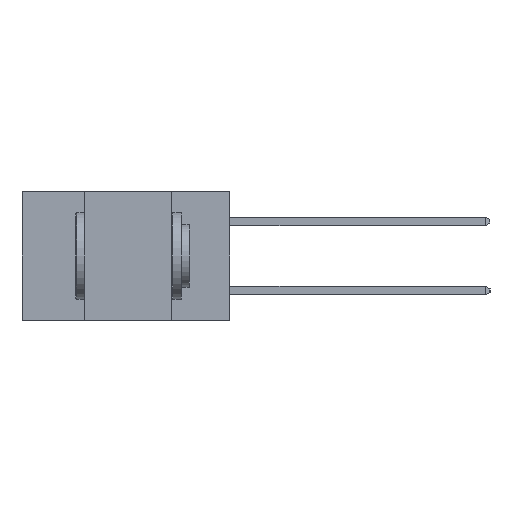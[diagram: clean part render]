
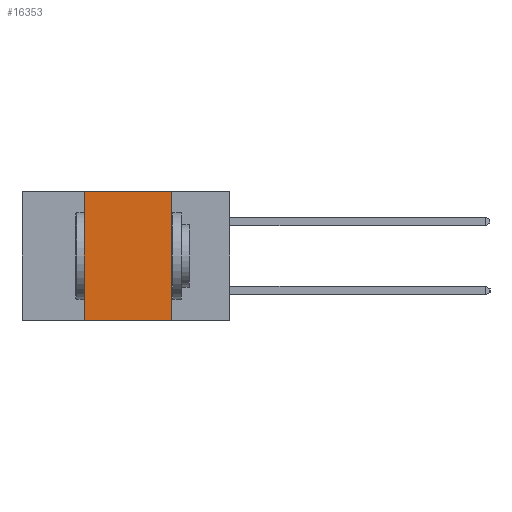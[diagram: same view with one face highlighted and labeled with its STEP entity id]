
A CAD part, left-side view. The second image highlights one B-rep face of the part: STEP entity #16353.
In plain terms, the highlighted planar face has unit normal (-1, 0, 0).
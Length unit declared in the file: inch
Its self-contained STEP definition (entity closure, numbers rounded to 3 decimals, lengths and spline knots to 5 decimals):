
#102 = VECTOR ( 'NONE', #20577, 39.37008 ) ;
#671 = ORIENTED_EDGE ( 'NONE', *, *, #18440, .T. ) ;
#1120 = DIRECTION ( 'NONE',  ( 0., -1., 0. ) ) ;
#3769 = ORIENTED_EDGE ( 'NONE', *, *, #21884, .F. ) ;
#5909 = FACE_OUTER_BOUND ( 'NONE', #11391, .T. ) ;
#6628 = CARTESIAN_POINT ( 'NONE',  ( 0., 0.6, 0. ) ) ;
#6913 = DIRECTION ( 'NONE',  ( 0., 0., 1. ) ) ;
#7944 = VERTEX_POINT ( 'NONE', #11834 ) ;
#8333 = VERTEX_POINT ( 'NONE', #8400 ) ;
#8400 = CARTESIAN_POINT ( 'NONE',  ( 0., 0.17, -0.37 ) ) ;
#8561 = VECTOR ( 'NONE', #1120, 39.37008 ) ;
#8564 = CARTESIAN_POINT ( 'NONE',  ( 0., 0.17, -0.37 ) ) ;
#9025 = ORIENTED_EDGE ( 'NONE', *, *, #19572, .F. ) ;
#9499 = DIRECTION ( 'NONE',  ( 0., 0., -1. ) ) ;
#11143 = PLANE ( 'NONE',  #19806 ) ;
#11391 = EDGE_LOOP ( 'NONE', ( #3769, #22169, #9025, #671 ) ) ;
#11834 = CARTESIAN_POINT ( 'NONE',  ( 0., 0.42, 0. ) ) ;
#12068 = LINE ( 'NONE', #21934, #8561 ) ;
#12415 = CARTESIAN_POINT ( 'NONE',  ( 0., 0.17, 0. ) ) ;
#12537 = LINE ( 'NONE', #13794, #16591 ) ;
#12584 = VERTEX_POINT ( 'NONE', #12415 ) ;
#13794 = CARTESIAN_POINT ( 'NONE',  ( 0., 0.42, -0.37 ) ) ;
#14913 = LINE ( 'NONE', #6628, #20034 ) ;
#16346 = CARTESIAN_POINT ( 'NONE',  ( 0., 0.6, 0. ) ) ;
#16353 = ADVANCED_FACE ( 'NONE', ( #5909 ), #11143, .F. ) ;
#16591 = VECTOR ( 'NONE', #6913, 39.37008 ) ;
#16983 = DIRECTION ( 'NONE',  ( 0., -1., 0. ) ) ;
#17008 = CARTESIAN_POINT ( 'NONE',  ( 0., 0.42, -0.37 ) ) ;
#18440 = EDGE_CURVE ( 'NONE', #20138, #8333, #12068, .T. ) ;
#19572 = EDGE_CURVE ( 'NONE', #20138, #7944, #12537, .T. ) ;
#19756 = DIRECTION ( 'NONE',  ( 1., 0., 0. ) ) ;
#19806 = AXIS2_PLACEMENT_3D ( 'NONE', #16346, #19756, #9499 ) ;
#20034 = VECTOR ( 'NONE', #16983, 39.37008 ) ;
#20138 = VERTEX_POINT ( 'NONE', #17008 ) ;
#20577 = DIRECTION ( 'NONE',  ( 0., 0., -1. ) ) ;
#20750 = EDGE_CURVE ( 'NONE', #7944, #12584, #14913, .T. ) ;
#21884 = EDGE_CURVE ( 'NONE', #12584, #8333, #22149, .T. ) ;
#21934 = CARTESIAN_POINT ( 'NONE',  ( 0., 0.6, -0.37 ) ) ;
#22149 = LINE ( 'NONE', #8564, #102 ) ;
#22169 = ORIENTED_EDGE ( 'NONE', *, *, #20750, .F. ) ;
